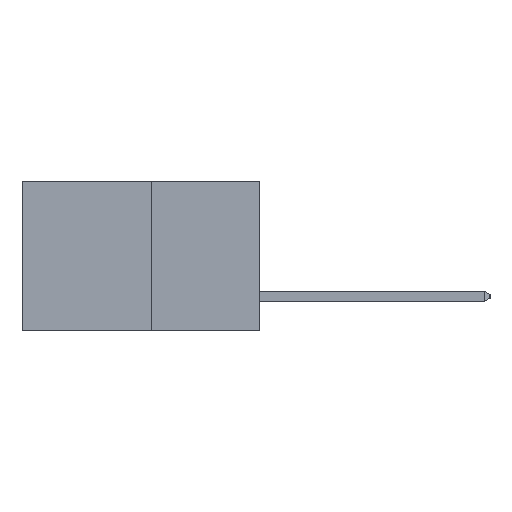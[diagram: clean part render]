
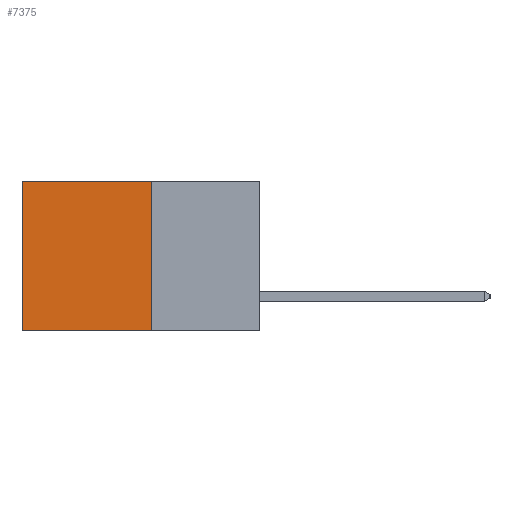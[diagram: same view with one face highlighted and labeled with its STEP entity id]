
A CAD part, left-side view. The second image highlights one B-rep face of the part: STEP entity #7375.
In plain terms, the highlighted planar face has unit normal (-1, 0, 0).
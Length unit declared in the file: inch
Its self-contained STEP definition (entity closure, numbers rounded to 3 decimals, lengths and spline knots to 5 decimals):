
#40 = VERTEX_POINT ( 'NONE', #10008 ) ;
#264 = VECTOR ( 'NONE', #8357, 39.37008 ) ;
#752 = CARTESIAN_POINT ( 'NONE',  ( 0.277, 0.27, 0. ) ) ;
#822 = EDGE_CURVE ( 'NONE', #10131, #5155, #4526, .T. ) ;
#963 = AXIS2_PLACEMENT_3D ( 'NONE', #8896, #3921, #9706 ) ;
#2154 = LINE ( 'NONE', #9568, #8289 ) ;
#2491 = CARTESIAN_POINT ( 'NONE',  ( 0.277, 0.59, 0. ) ) ;
#2597 = FACE_OUTER_BOUND ( 'NONE', #7855, .T. ) ;
#2623 = LINE ( 'NONE', #752, #264 ) ;
#3086 = CARTESIAN_POINT ( 'NONE',  ( 0.277, 0.27, -0.37 ) ) ;
#3089 = PLANE ( 'NONE',  #963 ) ;
#3831 = EDGE_CURVE ( 'NONE', #5155, #40, #2154, .T. ) ;
#3906 = EDGE_CURVE ( 'NONE', #4114, #40, #7541, .T. ) ;
#3921 = DIRECTION ( 'NONE',  ( 1., 0., 0. ) ) ;
#4114 = VERTEX_POINT ( 'NONE', #2491 ) ;
#4526 = LINE ( 'NONE', #10514, #8675 ) ;
#4687 = DIRECTION ( 'NONE',  ( 0., 0., -1. ) ) ;
#5155 = VERTEX_POINT ( 'NONE', #3086 ) ;
#5463 = DIRECTION ( 'NONE',  ( 0., 1., 0. ) ) ;
#5566 = CARTESIAN_POINT ( 'NONE',  ( 0.277, 0.59, -0.37 ) ) ;
#6127 = CARTESIAN_POINT ( 'NONE',  ( 0.277, 0.27, 0. ) ) ;
#6860 = DIRECTION ( 'NONE',  ( 0., 0., -1. ) ) ;
#7057 = ORIENTED_EDGE ( 'NONE', *, *, #3906, .T. ) ;
#7065 = ORIENTED_EDGE ( 'NONE', *, *, #10505, .T. ) ;
#7375 = ADVANCED_FACE ( 'NONE', ( #2597 ), #3089, .F. ) ;
#7541 = LINE ( 'NONE', #5566, #9433 ) ;
#7794 = ORIENTED_EDGE ( 'NONE', *, *, #3831, .F. ) ;
#7855 = EDGE_LOOP ( 'NONE', ( #7057, #7794, #8081, #7065 ) ) ;
#8081 = ORIENTED_EDGE ( 'NONE', *, *, #822, .F. ) ;
#8289 = VECTOR ( 'NONE', #5463, 39.37008 ) ;
#8357 = DIRECTION ( 'NONE',  ( 0., 1., 0. ) ) ;
#8675 = VECTOR ( 'NONE', #6860, 39.37008 ) ;
#8896 = CARTESIAN_POINT ( 'NONE',  ( 0.277, 0.27, -0.37 ) ) ;
#9433 = VECTOR ( 'NONE', #4687, 39.37008 ) ;
#9568 = CARTESIAN_POINT ( 'NONE',  ( 0.277, 0.27, -0.37 ) ) ;
#9706 = DIRECTION ( 'NONE',  ( 0., 0., -1. ) ) ;
#10008 = CARTESIAN_POINT ( 'NONE',  ( 0.277, 0.59, -0.37 ) ) ;
#10131 = VERTEX_POINT ( 'NONE', #6127 ) ;
#10505 = EDGE_CURVE ( 'NONE', #10131, #4114, #2623, .T. ) ;
#10514 = CARTESIAN_POINT ( 'NONE',  ( 0.277, 0.27, -0.37 ) ) ;
